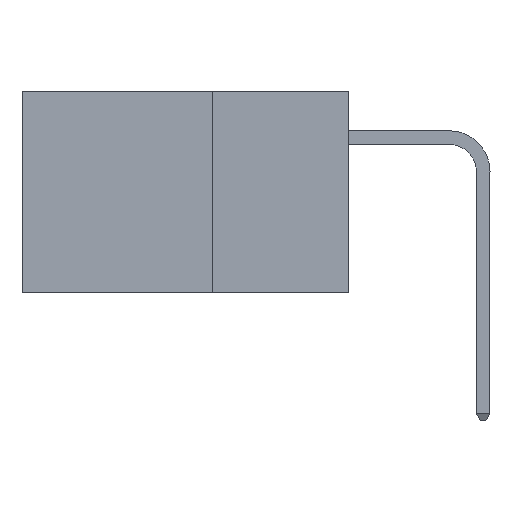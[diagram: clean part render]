
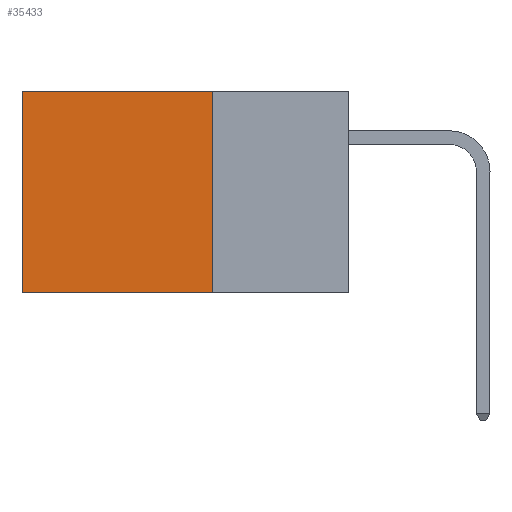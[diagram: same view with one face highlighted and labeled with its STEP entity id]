
A CAD part, left-side view. The second image highlights one B-rep face of the part: STEP entity #35433.
In plain terms, the highlighted planar face has unit normal (-1, 0, 0).
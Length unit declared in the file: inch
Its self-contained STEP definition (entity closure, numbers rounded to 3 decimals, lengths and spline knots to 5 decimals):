
#2290 = PLANE ( 'NONE',  #12122 ) ;
#2431 = VECTOR ( 'NONE', #32220, 39.37008 ) ;
#3253 = VERTEX_POINT ( 'NONE', #28229 ) ;
#5618 = CARTESIAN_POINT ( 'NONE',  ( 0.2875, 0.6, 0. ) ) ;
#8483 = VECTOR ( 'NONE', #11531, 39.37008 ) ;
#8921 = EDGE_CURVE ( 'NONE', #15934, #32597, #31471, .T. ) ;
#10794 = LINE ( 'NONE', #5618, #25980 ) ;
#11293 = FACE_OUTER_BOUND ( 'NONE', #33754, .T. ) ;
#11531 = DIRECTION ( 'NONE',  ( 0., 0., -1. ) ) ;
#12122 = AXIS2_PLACEMENT_3D ( 'NONE', #33993, #16858, #36808 ) ;
#13470 = ORIENTED_EDGE ( 'NONE', *, *, #32245, .T. ) ;
#15074 = CARTESIAN_POINT ( 'NONE',  ( 0.2875, 0.25, 0. ) ) ;
#15227 = LINE ( 'NONE', #28636, #8483 ) ;
#15431 = ORIENTED_EDGE ( 'NONE', *, *, #19992, .F. ) ;
#15934 = VERTEX_POINT ( 'NONE', #18050 ) ;
#16485 = CARTESIAN_POINT ( 'NONE',  ( 0.2875, 0.25, -0.37 ) ) ;
#16858 = DIRECTION ( 'NONE',  ( 1., 0., 0. ) ) ;
#17635 = VERTEX_POINT ( 'NONE', #26149 ) ;
#18050 = CARTESIAN_POINT ( 'NONE',  ( 0.2875, 0.25, -0.37 ) ) ;
#19331 = DIRECTION ( 'NONE',  ( 0., 1., 0. ) ) ;
#19992 = EDGE_CURVE ( 'NONE', #17635, #15934, #15227, .T. ) ;
#22907 = VECTOR ( 'NONE', #19331, 39.37008 ) ;
#25045 = ORIENTED_EDGE ( 'NONE', *, *, #30677, .T. ) ;
#25980 = VECTOR ( 'NONE', #34395, 39.37008 ) ;
#26149 = CARTESIAN_POINT ( 'NONE',  ( 0.2875, 0.25, 0. ) ) ;
#28229 = CARTESIAN_POINT ( 'NONE',  ( 0.2875, 0.6, 0. ) ) ;
#28636 = CARTESIAN_POINT ( 'NONE',  ( 0.2875, 0.25, 0. ) ) ;
#30677 = EDGE_CURVE ( 'NONE', #3253, #32597, #10794, .T. ) ;
#31471 = LINE ( 'NONE', #16485, #22907 ) ;
#32161 = LINE ( 'NONE', #15074, #2431 ) ;
#32188 = ORIENTED_EDGE ( 'NONE', *, *, #8921, .F. ) ;
#32220 = DIRECTION ( 'NONE',  ( 0., 1., 0. ) ) ;
#32245 = EDGE_CURVE ( 'NONE', #17635, #3253, #32161, .T. ) ;
#32597 = VERTEX_POINT ( 'NONE', #36629 ) ;
#33754 = EDGE_LOOP ( 'NONE', ( #25045, #32188, #15431, #13470 ) ) ;
#33993 = CARTESIAN_POINT ( 'NONE',  ( 0.2875, 0.25, 0. ) ) ;
#34395 = DIRECTION ( 'NONE',  ( 0., 0., -1. ) ) ;
#35433 = ADVANCED_FACE ( 'NONE', ( #11293 ), #2290, .F. ) ;
#36629 = CARTESIAN_POINT ( 'NONE',  ( 0.2875, 0.6, -0.37 ) ) ;
#36808 = DIRECTION ( 'NONE',  ( 0., 0., -1. ) ) ;
